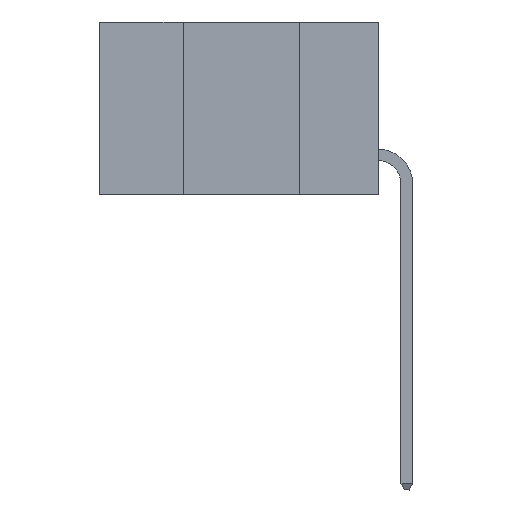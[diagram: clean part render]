
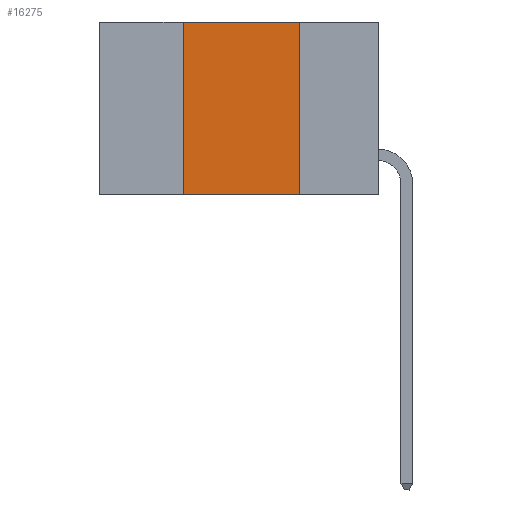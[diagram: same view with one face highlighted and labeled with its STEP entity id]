
A CAD part, left-side view. The second image highlights one B-rep face of the part: STEP entity #16275.
In plain terms, the highlighted planar face has unit normal (-1, 0, 0).
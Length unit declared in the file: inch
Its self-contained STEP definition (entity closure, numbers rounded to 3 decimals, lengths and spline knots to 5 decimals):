
#165 = CARTESIAN_POINT ( 'NONE',  ( 0., 0.42, -0.37 ) ) ;
#310 = FACE_OUTER_BOUND ( 'NONE', #16903, .T. ) ;
#438 = CARTESIAN_POINT ( 'NONE',  ( 0., 0.17, 0. ) ) ;
#495 = AXIS2_PLACEMENT_3D ( 'NONE', #8256, #5483, #13561 ) ;
#774 = ORIENTED_EDGE ( 'NONE', *, *, #16679, .T. ) ;
#2241 = ORIENTED_EDGE ( 'NONE', *, *, #11739, .F. ) ;
#2555 = CARTESIAN_POINT ( 'NONE',  ( 0., 0.17, -0.37 ) ) ;
#3571 = VECTOR ( 'NONE', #15720, 39.37008 ) ;
#3865 = CARTESIAN_POINT ( 'NONE',  ( 0., 0.6, -0.37 ) ) ;
#4195 = DIRECTION ( 'NONE',  ( 0., 0., 1. ) ) ;
#5483 = DIRECTION ( 'NONE',  ( 1., 0., 0. ) ) ;
#5689 = LINE ( 'NONE', #13427, #15409 ) ;
#5701 = VECTOR ( 'NONE', #4195, 39.37008 ) ;
#6986 = DIRECTION ( 'NONE',  ( 0., -1., 0. ) ) ;
#7042 = CARTESIAN_POINT ( 'NONE',  ( 0., 0.17, -0.37 ) ) ;
#8256 = CARTESIAN_POINT ( 'NONE',  ( 0., 0.6, 0. ) ) ;
#8366 = DIRECTION ( 'NONE',  ( 0., 0., -1. ) ) ;
#8490 = VERTEX_POINT ( 'NONE', #2555 ) ;
#9068 = EDGE_CURVE ( 'NONE', #17164, #16792, #5689, .T. ) ;
#10693 = PLANE ( 'NONE',  #495 ) ;
#11739 = EDGE_CURVE ( 'NONE', #16142, #17164, #13687, .T. ) ;
#12056 = LINE ( 'NONE', #3865, #3571 ) ;
#12271 = EDGE_CURVE ( 'NONE', #16792, #8490, #13850, .T. ) ;
#13138 = CARTESIAN_POINT ( 'NONE',  ( 0., 0.42, -0.37 ) ) ;
#13427 = CARTESIAN_POINT ( 'NONE',  ( 0., 0.6, 0. ) ) ;
#13432 = ORIENTED_EDGE ( 'NONE', *, *, #12271, .F. ) ;
#13561 = DIRECTION ( 'NONE',  ( 0., 0., -1. ) ) ;
#13687 = LINE ( 'NONE', #165, #5701 ) ;
#13850 = LINE ( 'NONE', #7042, #14619 ) ;
#14619 = VECTOR ( 'NONE', #8366, 39.37008 ) ;
#14900 = CARTESIAN_POINT ( 'NONE',  ( 0., 0.42, 0. ) ) ;
#15077 = ORIENTED_EDGE ( 'NONE', *, *, #9068, .F. ) ;
#15409 = VECTOR ( 'NONE', #6986, 39.37008 ) ;
#15720 = DIRECTION ( 'NONE',  ( 0., -1., 0. ) ) ;
#16142 = VERTEX_POINT ( 'NONE', #13138 ) ;
#16275 = ADVANCED_FACE ( 'NONE', ( #310 ), #10693, .F. ) ;
#16679 = EDGE_CURVE ( 'NONE', #16142, #8490, #12056, .T. ) ;
#16792 = VERTEX_POINT ( 'NONE', #438 ) ;
#16903 = EDGE_LOOP ( 'NONE', ( #13432, #15077, #2241, #774 ) ) ;
#17164 = VERTEX_POINT ( 'NONE', #14900 ) ;
